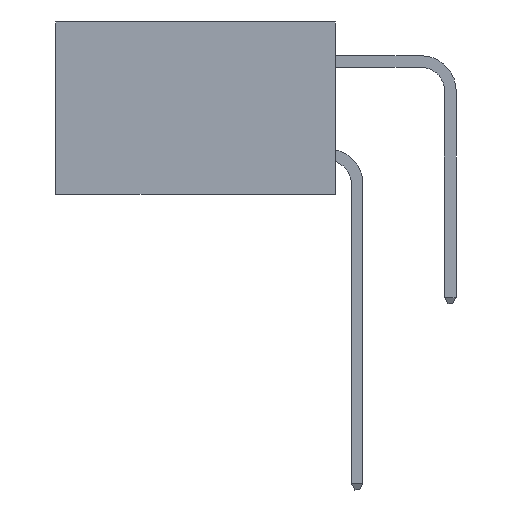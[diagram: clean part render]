
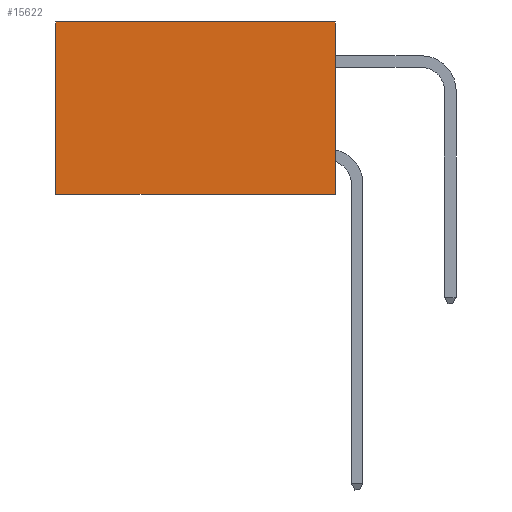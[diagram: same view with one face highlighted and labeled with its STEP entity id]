
A CAD part, left-side view. The second image highlights one B-rep face of the part: STEP entity #15622.
In plain terms, the highlighted planar face has unit normal (-1, 0, 0).
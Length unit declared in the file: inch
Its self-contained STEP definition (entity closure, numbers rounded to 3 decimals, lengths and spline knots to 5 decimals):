
#693 = DIRECTION ( 'NONE',  ( 0., 1., 0. ) ) ;
#2161 = CARTESIAN_POINT ( 'NONE',  ( 0.2875, 0.6, 0. ) ) ;
#2741 = DIRECTION ( 'NONE',  ( 1., 0., 0. ) ) ;
#2912 = VECTOR ( 'NONE', #693, 39.37008 ) ;
#3001 = VECTOR ( 'NONE', #21563, 39.37008 ) ;
#3555 = VERTEX_POINT ( 'NONE', #16519 ) ;
#3926 = VECTOR ( 'NONE', #18836, 39.37008 ) ;
#4187 = EDGE_CURVE ( 'NONE', #17730, #3555, #19868, .T. ) ;
#4508 = LINE ( 'NONE', #6455, #3926 ) ;
#5686 = EDGE_CURVE ( 'NONE', #9743, #3555, #4508, .T. ) ;
#6215 = PLANE ( 'NONE',  #8898 ) ;
#6455 = CARTESIAN_POINT ( 'NONE',  ( 0.2875, 0.6, 0. ) ) ;
#6612 = ORIENTED_EDGE ( 'NONE', *, *, #4187, .F. ) ;
#8609 = DIRECTION ( 'NONE',  ( 0., 0., -1. ) ) ;
#8885 = LINE ( 'NONE', #22375, #17960 ) ;
#8898 = AXIS2_PLACEMENT_3D ( 'NONE', #9954, #2741, #20251 ) ;
#9425 = ORIENTED_EDGE ( 'NONE', *, *, #20846, .F. ) ;
#9743 = VERTEX_POINT ( 'NONE', #2161 ) ;
#9954 = CARTESIAN_POINT ( 'NONE',  ( 0.2875, 0., 0. ) ) ;
#9956 = ORIENTED_EDGE ( 'NONE', *, *, #5686, .T. ) ;
#13052 = VERTEX_POINT ( 'NONE', #17935 ) ;
#13534 = FACE_OUTER_BOUND ( 'NONE', #21454, .T. ) ;
#15622 = ADVANCED_FACE ( 'NONE', ( #13534 ), #6215, .F. ) ;
#15644 = CARTESIAN_POINT ( 'NONE',  ( 0.2875, 0., -0.37 ) ) ;
#15867 = CARTESIAN_POINT ( 'NONE',  ( 0.2875, 0., 0. ) ) ;
#16131 = ORIENTED_EDGE ( 'NONE', *, *, #17776, .T. ) ;
#16519 = CARTESIAN_POINT ( 'NONE',  ( 0.2875, 0.6, -0.37 ) ) ;
#17730 = VERTEX_POINT ( 'NONE', #15644 ) ;
#17776 = EDGE_CURVE ( 'NONE', #13052, #9743, #17795, .T. ) ;
#17795 = LINE ( 'NONE', #15867, #3001 ) ;
#17935 = CARTESIAN_POINT ( 'NONE',  ( 0.2875, 0., 0. ) ) ;
#17960 = VECTOR ( 'NONE', #8609, 39.37008 ) ;
#18836 = DIRECTION ( 'NONE',  ( 0., 0., -1. ) ) ;
#19868 = LINE ( 'NONE', #21572, #2912 ) ;
#20251 = DIRECTION ( 'NONE',  ( 0., 0., -1. ) ) ;
#20846 = EDGE_CURVE ( 'NONE', #13052, #17730, #8885, .T. ) ;
#21454 = EDGE_LOOP ( 'NONE', ( #9956, #6612, #9425, #16131 ) ) ;
#21563 = DIRECTION ( 'NONE',  ( 0., 1., 0. ) ) ;
#21572 = CARTESIAN_POINT ( 'NONE',  ( 0.2875, 0., -0.37 ) ) ;
#22375 = CARTESIAN_POINT ( 'NONE',  ( 0.2875, 0., 0. ) ) ;
